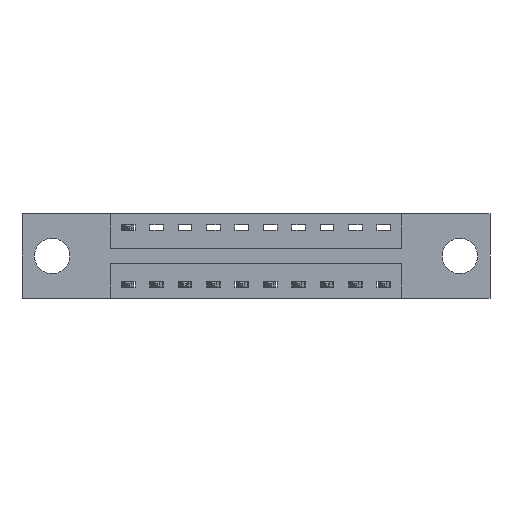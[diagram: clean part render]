
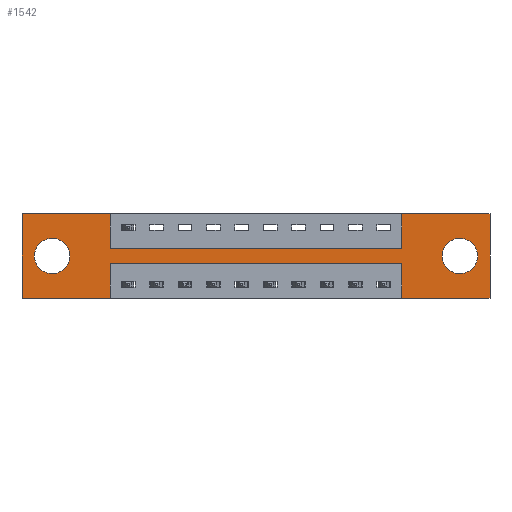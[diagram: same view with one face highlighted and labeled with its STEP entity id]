
A CAD part, front view. The second image highlights one B-rep face of the part: STEP entity #1542.
In plain terms, the highlighted planar face has unit normal (0, -1, 0).
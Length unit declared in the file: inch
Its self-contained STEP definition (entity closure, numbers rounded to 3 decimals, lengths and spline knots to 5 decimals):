
#158 = VECTOR ( 'NONE', #1380, 39.37008 ) ;
#170 = CIRCLE ( 'NONE', #2906, 0.078 ) ;
#171 = VECTOR ( 'NONE', #4387, 39.37008 ) ;
#183 = CARTESIAN_POINT ( 'NONE',  ( 0.1325, 0., -0.263 ) ) ;
#196 = DIRECTION ( 'NONE',  ( 0., 1., 0. ) ) ;
#464 = ORIENTED_EDGE ( 'NONE', *, *, #5562, .F. ) ;
#637 = CARTESIAN_POINT ( 'NONE',  ( 2.06, 0., 0. ) ) ;
#671 = LINE ( 'NONE', #8849, #2449 ) ;
#698 = VERTEX_POINT ( 'NONE', #3492 ) ;
#733 = DIRECTION ( 'NONE',  ( -1., 0., 0. ) ) ;
#836 = VERTEX_POINT ( 'NONE', #8749 ) ;
#862 = VERTEX_POINT ( 'NONE', #2150 ) ;
#1380 = DIRECTION ( 'NONE',  ( 0., 0., -1. ) ) ;
#1542 = ADVANCED_FACE ( 'NONE', ( #6710, #2407, #2923 ), #8192, .T. ) ;
#1710 = CARTESIAN_POINT ( 'NONE',  ( 0., 0., 0. ) ) ;
#1735 = CARTESIAN_POINT ( 'NONE',  ( 2.06, 0., 0. ) ) ;
#1751 = LINE ( 'NONE', #1735, #5830 ) ;
#1760 = VECTOR ( 'NONE', #5273, 39.37008 ) ;
#1767 = DIRECTION ( 'NONE',  ( 0., -1., 0. ) ) ;
#1820 = CARTESIAN_POINT ( 'NONE',  ( 0., 0., 0. ) ) ;
#1978 = CARTESIAN_POINT ( 'NONE',  ( 1.9275, 0., -0.185 ) ) ;
#2150 = CARTESIAN_POINT ( 'NONE',  ( 0.3875, 0., -0.15 ) ) ;
#2166 = ORIENTED_EDGE ( 'NONE', *, *, #9579, .F. ) ;
#2223 = EDGE_CURVE ( 'NONE', #8507, #4258, #10479, .T. ) ;
#2261 = CARTESIAN_POINT ( 'NONE',  ( 1.6725, 0., -0.15 ) ) ;
#2397 = LINE ( 'NONE', #1710, #9021 ) ;
#2407 = FACE_BOUND ( 'NONE', #6001, .T. ) ;
#2443 = LINE ( 'NONE', #8616, #8578 ) ;
#2449 = VECTOR ( 'NONE', #733, 39.37008 ) ;
#2640 = EDGE_CURVE ( 'NONE', #5102, #5006, #170, .T. ) ;
#2775 = DIRECTION ( 'NONE',  ( 0., 0., -1. ) ) ;
#2790 = ORIENTED_EDGE ( 'NONE', *, *, #8931, .F. ) ;
#2906 = AXIS2_PLACEMENT_3D ( 'NONE', #1978, #7586, #2775 ) ;
#2923 = FACE_OUTER_BOUND ( 'NONE', #7909, .T. ) ;
#3064 = EDGE_CURVE ( 'NONE', #10242, #862, #6821, .T. ) ;
#3072 = CARTESIAN_POINT ( 'NONE',  ( 0.3875, 0., 0. ) ) ;
#3135 = CARTESIAN_POINT ( 'NONE',  ( 0.3875, 0., -0.15 ) ) ;
#3422 = CARTESIAN_POINT ( 'NONE',  ( 0.3875, 0., 0. ) ) ;
#3492 = CARTESIAN_POINT ( 'NONE',  ( 2.06, 0., -0.37 ) ) ;
#3610 = VECTOR ( 'NONE', #7152, 39.37008 ) ;
#3868 = LINE ( 'NONE', #3135, #3610 ) ;
#3939 = LINE ( 'NONE', #8408, #1760 ) ;
#3940 = ORIENTED_EDGE ( 'NONE', *, *, #7631, .T. ) ;
#3958 = VERTEX_POINT ( 'NONE', #637 ) ;
#4214 = CARTESIAN_POINT ( 'NONE',  ( 1.9275, 0., -0.263 ) ) ;
#4258 = VERTEX_POINT ( 'NONE', #4296 ) ;
#4272 = CARTESIAN_POINT ( 'NONE',  ( 0.1325, 0., -0.185 ) ) ;
#4296 = CARTESIAN_POINT ( 'NONE',  ( 0.3875, 0., -0.37 ) ) ;
#4387 = DIRECTION ( 'NONE',  ( -1., 0., 0. ) ) ;
#4826 = CARTESIAN_POINT ( 'NONE',  ( 0.1325, 0., -0.185 ) ) ;
#4872 = EDGE_CURVE ( 'NONE', #4258, #6178, #671, .T. ) ;
#4874 = DIRECTION ( 'NONE',  ( 0., 0., 1. ) ) ;
#4888 = CARTESIAN_POINT ( 'NONE',  ( 0.3875, 0., -0.22 ) ) ;
#4940 = ORIENTED_EDGE ( 'NONE', *, *, #3064, .F. ) ;
#5006 = VERTEX_POINT ( 'NONE', #4214 ) ;
#5084 = DIRECTION ( 'NONE',  ( 0., 0., 1. ) ) ;
#5102 = VERTEX_POINT ( 'NONE', #5910 ) ;
#5201 = LINE ( 'NONE', #8803, #8883 ) ;
#5261 = CARTESIAN_POINT ( 'NONE',  ( 1.9275, 0., -0.185 ) ) ;
#5273 = DIRECTION ( 'NONE',  ( 0., 0., 1. ) ) ;
#5311 = CIRCLE ( 'NONE', #6570, 0.078 ) ;
#5339 = VECTOR ( 'NONE', #10572, 39.37008 ) ;
#5413 = VERTEX_POINT ( 'NONE', #10075 ) ;
#5476 = DIRECTION ( 'NONE',  ( -1., 0., 0. ) ) ;
#5492 = EDGE_CURVE ( 'NONE', #5413, #8507, #2443, .T. ) ;
#5503 = CARTESIAN_POINT ( 'NONE',  ( 0., 0., -0.37 ) ) ;
#5528 = CARTESIAN_POINT ( 'NONE',  ( 0.1325, 0., -0.107 ) ) ;
#5548 = CARTESIAN_POINT ( 'NONE',  ( 0.3875, 0., -0.37 ) ) ;
#5562 = EDGE_CURVE ( 'NONE', #862, #7496, #3868, .T. ) ;
#5644 = DIRECTION ( 'NONE',  ( 0., 0., 1. ) ) ;
#5718 = ORIENTED_EDGE ( 'NONE', *, *, #9435, .F. ) ;
#5780 = DIRECTION ( 'NONE',  ( 1., 0., 0. ) ) ;
#5827 = CARTESIAN_POINT ( 'NONE',  ( 0., 0., -0.37 ) ) ;
#5830 = VECTOR ( 'NONE', #7379, 39.37008 ) ;
#5910 = CARTESIAN_POINT ( 'NONE',  ( 1.9275, 0., -0.107 ) ) ;
#6001 = EDGE_LOOP ( 'NONE', ( #3940, #10235 ) ) ;
#6072 = DIRECTION ( 'NONE',  ( 0., 0., -1. ) ) ;
#6178 = VERTEX_POINT ( 'NONE', #5503 ) ;
#6195 = CIRCLE ( 'NONE', #8672, 0.078 ) ;
#6227 = ORIENTED_EDGE ( 'NONE', *, *, #8584, .F. ) ;
#6325 = ORIENTED_EDGE ( 'NONE', *, *, #5492, .F. ) ;
#6332 = VECTOR ( 'NONE', #6355, 39.37008 ) ;
#6355 = DIRECTION ( 'NONE',  ( 0., 0., -1. ) ) ;
#6570 = AXIS2_PLACEMENT_3D ( 'NONE', #4272, #9773, #5084 ) ;
#6571 = LINE ( 'NONE', #9897, #171 ) ;
#6573 = ORIENTED_EDGE ( 'NONE', *, *, #9899, .F. ) ;
#6710 = FACE_BOUND ( 'NONE', #8685, .T. ) ;
#6821 = LINE ( 'NONE', #3072, #158 ) ;
#6830 = DIRECTION ( 'NONE',  ( 0., 0., 1. ) ) ;
#6831 = ORIENTED_EDGE ( 'NONE', *, *, #2223, .F. ) ;
#6990 = EDGE_CURVE ( 'NONE', #836, #10242, #7451, .T. ) ;
#7081 = ORIENTED_EDGE ( 'NONE', *, *, #4872, .F. ) ;
#7152 = DIRECTION ( 'NONE',  ( 1., 0., 0. ) ) ;
#7379 = DIRECTION ( 'NONE',  ( 0., 0., -1. ) ) ;
#7451 = LINE ( 'NONE', #1820, #5339 ) ;
#7496 = VERTEX_POINT ( 'NONE', #2261 ) ;
#7566 = ORIENTED_EDGE ( 'NONE', *, *, #6990, .F. ) ;
#7586 = DIRECTION ( 'NONE',  ( 0., 1., 0. ) ) ;
#7631 = EDGE_CURVE ( 'NONE', #8295, #8042, #9624, .T. ) ;
#7909 = EDGE_LOOP ( 'NONE', ( #6831, #6325, #6573, #10471, #2166, #6227, #2790, #464, #4940, #7566, #5718, #7081 ) ) ;
#7964 = CARTESIAN_POINT ( 'NONE',  ( 1.6725, 0., -0.37 ) ) ;
#8042 = VERTEX_POINT ( 'NONE', #183 ) ;
#8057 = AXIS2_PLACEMENT_3D ( 'NONE', #5827, #1767, #9731 ) ;
#8192 = PLANE ( 'NONE',  #8057 ) ;
#8295 = VERTEX_POINT ( 'NONE', #5528 ) ;
#8408 = CARTESIAN_POINT ( 'NONE',  ( 1.6725, 0., 0. ) ) ;
#8507 = VERTEX_POINT ( 'NONE', #4888 ) ;
#8578 = VECTOR ( 'NONE', #5476, 39.37008 ) ;
#8584 = EDGE_CURVE ( 'NONE', #8779, #3958, #2397, .T. ) ;
#8616 = CARTESIAN_POINT ( 'NONE',  ( 0.3875, 0., -0.22 ) ) ;
#8656 = ORIENTED_EDGE ( 'NONE', *, *, #2640, .T. ) ;
#8672 = AXIS2_PLACEMENT_3D ( 'NONE', #5261, #196, #6072 ) ;
#8685 = EDGE_LOOP ( 'NONE', ( #8656, #8891 ) ) ;
#8749 = CARTESIAN_POINT ( 'NONE',  ( 0., 0., 0. ) ) ;
#8779 = VERTEX_POINT ( 'NONE', #9056 ) ;
#8803 = CARTESIAN_POINT ( 'NONE',  ( 0., 0., 0. ) ) ;
#8849 = CARTESIAN_POINT ( 'NONE',  ( 0., 0., -0.37 ) ) ;
#8868 = EDGE_CURVE ( 'NONE', #698, #9323, #6571, .T. ) ;
#8883 = VECTOR ( 'NONE', #4874, 39.37008 ) ;
#8891 = ORIENTED_EDGE ( 'NONE', *, *, #9894, .T. ) ;
#8931 = EDGE_CURVE ( 'NONE', #7496, #8779, #3939, .T. ) ;
#9021 = VECTOR ( 'NONE', #5780, 39.37008 ) ;
#9056 = CARTESIAN_POINT ( 'NONE',  ( 1.6725, 0., 0. ) ) ;
#9323 = VERTEX_POINT ( 'NONE', #7964 ) ;
#9435 = EDGE_CURVE ( 'NONE', #6178, #836, #5201, .T. ) ;
#9552 = AXIS2_PLACEMENT_3D ( 'NONE', #4826, #10320, #5644 ) ;
#9579 = EDGE_CURVE ( 'NONE', #3958, #698, #1751, .T. ) ;
#9624 = CIRCLE ( 'NONE', #9552, 0.078 ) ;
#9673 = EDGE_CURVE ( 'NONE', #8042, #8295, #5311, .T. ) ;
#9731 = DIRECTION ( 'NONE',  ( 0., 0., -1. ) ) ;
#9773 = DIRECTION ( 'NONE',  ( 0., 1., 0. ) ) ;
#9839 = VECTOR ( 'NONE', #6830, 39.37008 ) ;
#9894 = EDGE_CURVE ( 'NONE', #5006, #5102, #6195, .T. ) ;
#9897 = CARTESIAN_POINT ( 'NONE',  ( 0., 0., -0.37 ) ) ;
#9899 = EDGE_CURVE ( 'NONE', #9323, #5413, #10103, .T. ) ;
#9951 = CARTESIAN_POINT ( 'NONE',  ( 1.6725, 0., -0.37 ) ) ;
#10075 = CARTESIAN_POINT ( 'NONE',  ( 1.6725, 0., -0.22 ) ) ;
#10103 = LINE ( 'NONE', #9951, #9839 ) ;
#10235 = ORIENTED_EDGE ( 'NONE', *, *, #9673, .T. ) ;
#10242 = VERTEX_POINT ( 'NONE', #3422 ) ;
#10320 = DIRECTION ( 'NONE',  ( 0., 1., 0. ) ) ;
#10471 = ORIENTED_EDGE ( 'NONE', *, *, #8868, .F. ) ;
#10479 = LINE ( 'NONE', #5548, #6332 ) ;
#10572 = DIRECTION ( 'NONE',  ( 1., 0., 0. ) ) ;
